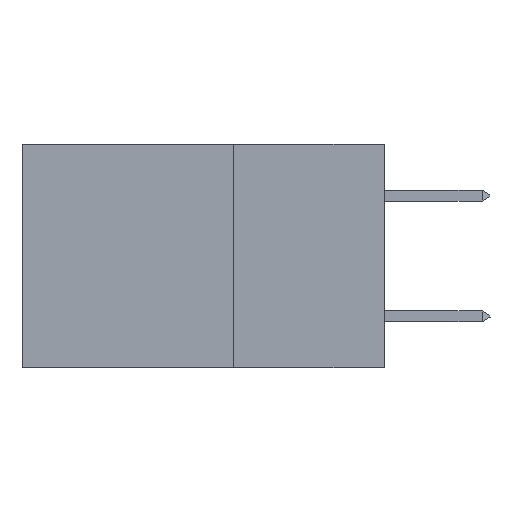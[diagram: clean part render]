
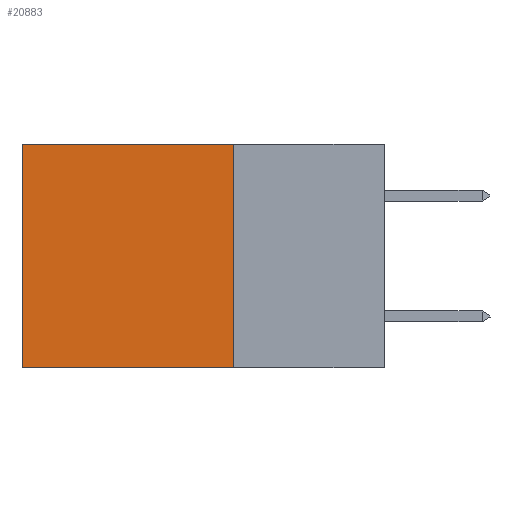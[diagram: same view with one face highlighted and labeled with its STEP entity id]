
A CAD part, left-side view. The second image highlights one B-rep face of the part: STEP entity #20883.
In plain terms, the highlighted planar face has unit normal (-1, 0, 0).
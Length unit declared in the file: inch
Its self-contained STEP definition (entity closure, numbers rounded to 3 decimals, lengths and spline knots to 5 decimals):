
#127 = VERTEX_POINT ( 'NONE', #19495 ) ;
#1182 = VECTOR ( 'NONE', #21431, 39.37008 ) ;
#1655 = ORIENTED_EDGE ( 'NONE', *, *, #2042, .F. ) ;
#1982 = VERTEX_POINT ( 'NONE', #22448 ) ;
#2042 = EDGE_CURVE ( 'NONE', #17969, #1982, #21313, .T. ) ;
#2313 = LINE ( 'NONE', #18354, #1182 ) ;
#4025 = CARTESIAN_POINT ( 'NONE',  ( 0.2875, 0.25, 0. ) ) ;
#5221 = ORIENTED_EDGE ( 'NONE', *, *, #9164, .F. ) ;
#5519 = CARTESIAN_POINT ( 'NONE',  ( 0.2875, 0.25, 0. ) ) ;
#5845 = DIRECTION ( 'NONE',  ( 0., 0., -1. ) ) ;
#6856 = DIRECTION ( 'NONE',  ( 0., 0., -1. ) ) ;
#7351 = EDGE_CURVE ( 'NONE', #17969, #15547, #2313, .T. ) ;
#7875 = VECTOR ( 'NONE', #5845, 39.37008 ) ;
#7980 = DIRECTION ( 'NONE',  ( 1., 0., 0. ) ) ;
#8461 = CARTESIAN_POINT ( 'NONE',  ( 0.2875, 0.6, 0. ) ) ;
#9050 = DIRECTION ( 'NONE',  ( 0., 0., -1. ) ) ;
#9164 = EDGE_CURVE ( 'NONE', #1982, #127, #20221, .T. ) ;
#9463 = VECTOR ( 'NONE', #13067, 39.37008 ) ;
#10251 = VECTOR ( 'NONE', #6856, 39.37008 ) ;
#13067 = DIRECTION ( 'NONE',  ( 0., 1., 0. ) ) ;
#15547 = VERTEX_POINT ( 'NONE', #8461 ) ;
#16074 = AXIS2_PLACEMENT_3D ( 'NONE', #5519, #7980, #9050 ) ;
#16867 = CARTESIAN_POINT ( 'NONE',  ( 0.2875, 0.6, 0. ) ) ;
#16985 = LINE ( 'NONE', #16867, #10251 ) ;
#17440 = EDGE_LOOP ( 'NONE', ( #21020, #5221, #1655, #20009 ) ) ;
#17969 = VERTEX_POINT ( 'NONE', #22202 ) ;
#18354 = CARTESIAN_POINT ( 'NONE',  ( 0.2875, 0.25, 0. ) ) ;
#19293 = EDGE_CURVE ( 'NONE', #15547, #127, #16985, .T. ) ;
#19495 = CARTESIAN_POINT ( 'NONE',  ( 0.2875, 0.6, -0.37 ) ) ;
#19516 = PLANE ( 'NONE',  #16074 ) ;
#20009 = ORIENTED_EDGE ( 'NONE', *, *, #7351, .T. ) ;
#20158 = FACE_OUTER_BOUND ( 'NONE', #17440, .T. ) ;
#20221 = LINE ( 'NONE', #21596, #9463 ) ;
#20883 = ADVANCED_FACE ( 'NONE', ( #20158 ), #19516, .F. ) ;
#21020 = ORIENTED_EDGE ( 'NONE', *, *, #19293, .T. ) ;
#21313 = LINE ( 'NONE', #4025, #7875 ) ;
#21431 = DIRECTION ( 'NONE',  ( 0., 1., 0. ) ) ;
#21596 = CARTESIAN_POINT ( 'NONE',  ( 0.2875, 0.25, -0.37 ) ) ;
#22202 = CARTESIAN_POINT ( 'NONE',  ( 0.2875, 0.25, 0. ) ) ;
#22448 = CARTESIAN_POINT ( 'NONE',  ( 0.2875, 0.25, -0.37 ) ) ;
